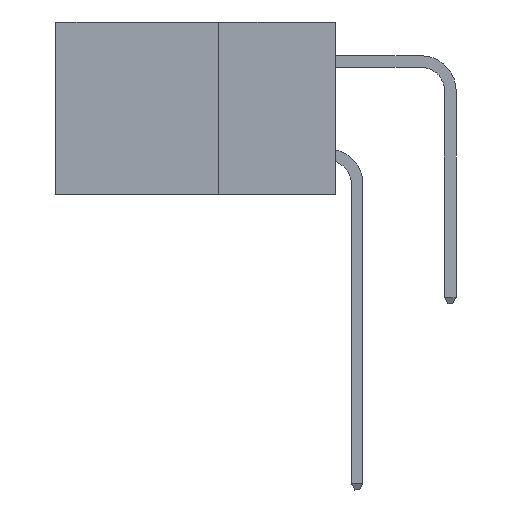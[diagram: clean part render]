
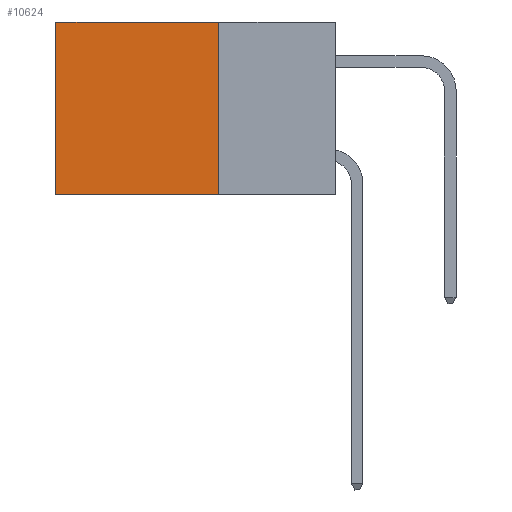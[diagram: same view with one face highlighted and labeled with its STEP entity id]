
A CAD part, left-side view. The second image highlights one B-rep face of the part: STEP entity #10624.
In plain terms, the highlighted planar face has unit normal (-1, 0, 0).
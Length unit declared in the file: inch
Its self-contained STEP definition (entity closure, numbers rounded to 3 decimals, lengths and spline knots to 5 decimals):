
#630 = VECTOR ( 'NONE', #28055, 39.37008 ) ;
#2399 = VERTEX_POINT ( 'NONE', #21665 ) ;
#2457 = CARTESIAN_POINT ( 'NONE',  ( 0.2875, 0.6, -0.37 ) ) ;
#2663 = LINE ( 'NONE', #14378, #5553 ) ;
#4281 = LINE ( 'NONE', #12231, #9290 ) ;
#4938 = ORIENTED_EDGE ( 'NONE', *, *, #4992, .F. ) ;
#4992 = EDGE_CURVE ( 'NONE', #24582, #15163, #4281, .T. ) ;
#5553 = VECTOR ( 'NONE', #13312, 39.37008 ) ;
#6464 = EDGE_CURVE ( 'NONE', #2399, #7389, #11737, .T. ) ;
#7028 = DIRECTION ( 'NONE',  ( 0., 0., -1. ) ) ;
#7389 = VERTEX_POINT ( 'NONE', #2457 ) ;
#9290 = VECTOR ( 'NONE', #22980, 39.37008 ) ;
#9799 = EDGE_CURVE ( 'NONE', #24582, #2399, #14894, .T. ) ;
#10624 = ADVANCED_FACE ( 'NONE', ( #18953 ), #22735, .F. ) ;
#10759 = EDGE_CURVE ( 'NONE', #15163, #7389, #2663, .T. ) ;
#10966 = DIRECTION ( 'NONE',  ( 0., 0., -1. ) ) ;
#11737 = LINE ( 'NONE', #32356, #12128 ) ;
#12128 = VECTOR ( 'NONE', #10966, 39.37008 ) ;
#12231 = CARTESIAN_POINT ( 'NONE',  ( 0.2875, 0.25, 0. ) ) ;
#13312 = DIRECTION ( 'NONE',  ( 0., 1., 0. ) ) ;
#13828 = EDGE_LOOP ( 'NONE', ( #22471, #21694, #4938, #17025 ) ) ;
#14378 = CARTESIAN_POINT ( 'NONE',  ( 0.2875, 0.25, -0.37 ) ) ;
#14616 = CARTESIAN_POINT ( 'NONE',  ( 0.2875, 0.25, 0. ) ) ;
#14830 = CARTESIAN_POINT ( 'NONE',  ( 0.2875, 0.25, 0. ) ) ;
#14894 = LINE ( 'NONE', #14616, #630 ) ;
#15088 = AXIS2_PLACEMENT_3D ( 'NONE', #28238, #33695, #7028 ) ;
#15163 = VERTEX_POINT ( 'NONE', #16488 ) ;
#16488 = CARTESIAN_POINT ( 'NONE',  ( 0.2875, 0.25, -0.37 ) ) ;
#17025 = ORIENTED_EDGE ( 'NONE', *, *, #9799, .T. ) ;
#18953 = FACE_OUTER_BOUND ( 'NONE', #13828, .T. ) ;
#21665 = CARTESIAN_POINT ( 'NONE',  ( 0.2875, 0.6, 0. ) ) ;
#21694 = ORIENTED_EDGE ( 'NONE', *, *, #10759, .F. ) ;
#22471 = ORIENTED_EDGE ( 'NONE', *, *, #6464, .T. ) ;
#22735 = PLANE ( 'NONE',  #15088 ) ;
#22980 = DIRECTION ( 'NONE',  ( 0., 0., -1. ) ) ;
#24582 = VERTEX_POINT ( 'NONE', #14830 ) ;
#28055 = DIRECTION ( 'NONE',  ( 0., 1., 0. ) ) ;
#28238 = CARTESIAN_POINT ( 'NONE',  ( 0.2875, 0.25, 0. ) ) ;
#32356 = CARTESIAN_POINT ( 'NONE',  ( 0.2875, 0.6, 0. ) ) ;
#33695 = DIRECTION ( 'NONE',  ( 1., 0., 0. ) ) ;
